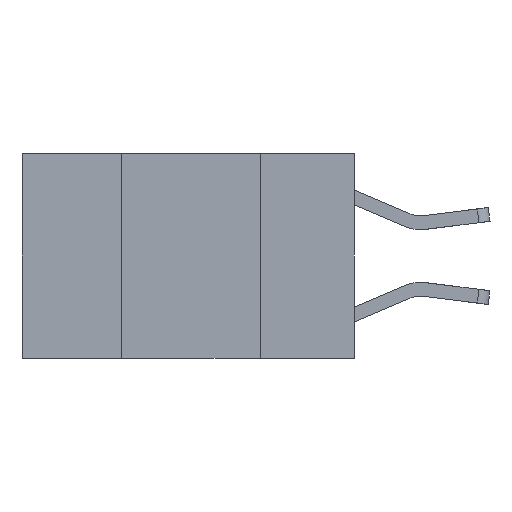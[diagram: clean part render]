
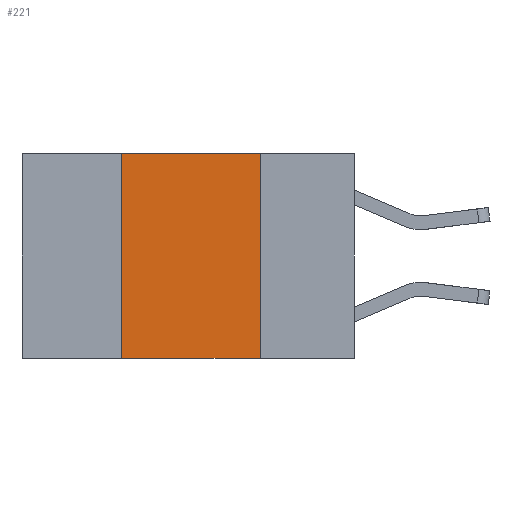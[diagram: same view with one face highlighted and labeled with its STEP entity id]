
A CAD part, left-side view. The second image highlights one B-rep face of the part: STEP entity #221.
In plain terms, the highlighted planar face has unit normal (-1, 0, 0).
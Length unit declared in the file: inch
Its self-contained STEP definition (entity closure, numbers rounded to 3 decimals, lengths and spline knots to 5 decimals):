
#63 = VECTOR ( 'NONE', #5575, 39.37008 ) ;
#221 = ADVANCED_FACE ( 'NONE', ( #10008 ), #7643, .F. ) ;
#329 = ORIENTED_EDGE ( 'NONE', *, *, #4129, .F. ) ;
#422 = DIRECTION ( 'NONE',  ( 0., 0., -1. ) ) ;
#576 = LINE ( 'NONE', #3883, #63 ) ;
#591 = AXIS2_PLACEMENT_3D ( 'NONE', #3543, #10229, #2850 ) ;
#820 = CARTESIAN_POINT ( 'NONE',  ( 0., 0.6, -0.37 ) ) ;
#862 = ORIENTED_EDGE ( 'NONE', *, *, #9030, .F. ) ;
#1189 = VERTEX_POINT ( 'NONE', #10069 ) ;
#1875 = DIRECTION ( 'NONE',  ( 0., -1., 0. ) ) ;
#2838 = CARTESIAN_POINT ( 'NONE',  ( 0., 0.6, 0. ) ) ;
#2850 = DIRECTION ( 'NONE',  ( 0., 0., -1. ) ) ;
#3222 = ORIENTED_EDGE ( 'NONE', *, *, #10246, .T. ) ;
#3333 = VECTOR ( 'NONE', #1875, 39.37008 ) ;
#3543 = CARTESIAN_POINT ( 'NONE',  ( 0., 0.6, 0. ) ) ;
#3616 = CARTESIAN_POINT ( 'NONE',  ( 0., 0.42, 0. ) ) ;
#3651 = VERTEX_POINT ( 'NONE', #7943 ) ;
#3883 = CARTESIAN_POINT ( 'NONE',  ( 0., 0.42, 0. ) ) ;
#4021 = LINE ( 'NONE', #820, #4081 ) ;
#4081 = VECTOR ( 'NONE', #4134, 39.37008 ) ;
#4129 = EDGE_CURVE ( 'NONE', #9859, #3651, #5112, .T. ) ;
#4134 = DIRECTION ( 'NONE',  ( 0., -1., 0. ) ) ;
#4200 = VECTOR ( 'NONE', #422, 39.37008 ) ;
#4393 = EDGE_CURVE ( 'NONE', #3651, #7410, #7134, .T. ) ;
#4519 = EDGE_LOOP ( 'NONE', ( #9340, #329, #862, #3222 ) ) ;
#5035 = CARTESIAN_POINT ( 'NONE',  ( 0., 0.17, -0.37 ) ) ;
#5112 = LINE ( 'NONE', #2838, #3333 ) ;
#5575 = DIRECTION ( 'NONE',  ( 0., 0., 1. ) ) ;
#7134 = LINE ( 'NONE', #10424, #4200 ) ;
#7410 = VERTEX_POINT ( 'NONE', #5035 ) ;
#7643 = PLANE ( 'NONE',  #591 ) ;
#7943 = CARTESIAN_POINT ( 'NONE',  ( 0., 0.17, 0. ) ) ;
#9030 = EDGE_CURVE ( 'NONE', #1189, #9859, #576, .T. ) ;
#9340 = ORIENTED_EDGE ( 'NONE', *, *, #4393, .F. ) ;
#9859 = VERTEX_POINT ( 'NONE', #3616 ) ;
#10008 = FACE_OUTER_BOUND ( 'NONE', #4519, .T. ) ;
#10069 = CARTESIAN_POINT ( 'NONE',  ( 0., 0.42, -0.37 ) ) ;
#10229 = DIRECTION ( 'NONE',  ( 1., 0., 0. ) ) ;
#10246 = EDGE_CURVE ( 'NONE', #1189, #7410, #4021, .T. ) ;
#10424 = CARTESIAN_POINT ( 'NONE',  ( 0., 0.17, 0. ) ) ;
